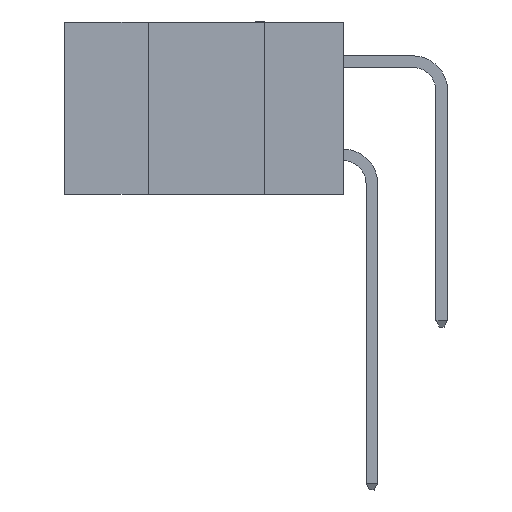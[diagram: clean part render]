
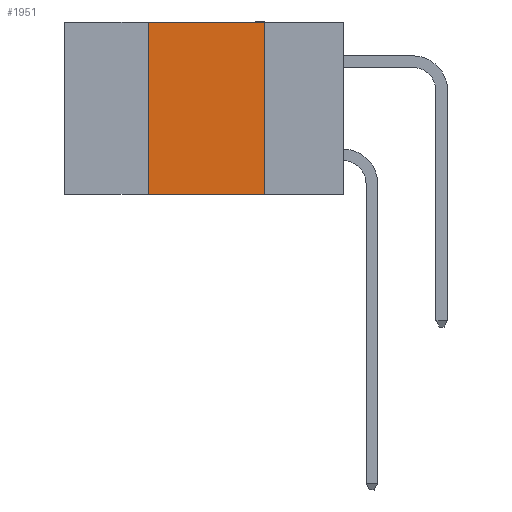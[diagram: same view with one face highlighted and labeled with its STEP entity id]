
A CAD part, left-side view. The second image highlights one B-rep face of the part: STEP entity #1951.
In plain terms, the highlighted planar face has unit normal (-1, 0, 0).
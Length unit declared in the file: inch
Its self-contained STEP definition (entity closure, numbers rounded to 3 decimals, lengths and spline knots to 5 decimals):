
#231 = CARTESIAN_POINT ( 'NONE',  ( 0., 0.42, -0.37 ) ) ;
#1951 = ADVANCED_FACE ( 'NONE', ( #21631 ), #26591, .F. ) ;
#3269 = DIRECTION ( 'NONE',  ( 1., 0., 0. ) ) ;
#3896 = EDGE_CURVE ( 'NONE', #22698, #11320, #11209, .T. ) ;
#4561 = ORIENTED_EDGE ( 'NONE', *, *, #11074, .F. ) ;
#5219 = DIRECTION ( 'NONE',  ( 0., 0., -1. ) ) ;
#5427 = DIRECTION ( 'NONE',  ( 0., 0., -1. ) ) ;
#6003 = CARTESIAN_POINT ( 'NONE',  ( 0., 0.17, -0.37 ) ) ;
#6651 = ORIENTED_EDGE ( 'NONE', *, *, #8108, .F. ) ;
#7099 = LINE ( 'NONE', #7462, #9716 ) ;
#7162 = ORIENTED_EDGE ( 'NONE', *, *, #3896, .T. ) ;
#7462 = CARTESIAN_POINT ( 'NONE',  ( 0., 0.6, 0. ) ) ;
#8108 = EDGE_CURVE ( 'NONE', #22698, #24449, #14214, .T. ) ;
#9568 = DIRECTION ( 'NONE',  ( 0., -1., 0. ) ) ;
#9716 = VECTOR ( 'NONE', #9568, 39.37008 ) ;
#10624 = VECTOR ( 'NONE', #5427, 39.37008 ) ;
#10855 = CARTESIAN_POINT ( 'NONE',  ( 0., 0.6, -0.37 ) ) ;
#11074 = EDGE_CURVE ( 'NONE', #24449, #17799, #7099, .T. ) ;
#11209 = LINE ( 'NONE', #10855, #22180 ) ;
#11320 = VERTEX_POINT ( 'NONE', #6003 ) ;
#11973 = CARTESIAN_POINT ( 'NONE',  ( 0., 0.17, 0. ) ) ;
#12795 = EDGE_LOOP ( 'NONE', ( #14413, #4561, #6651, #7162 ) ) ;
#13287 = LINE ( 'NONE', #11973, #10624 ) ;
#14214 = LINE ( 'NONE', #14961, #22496 ) ;
#14413 = ORIENTED_EDGE ( 'NONE', *, *, #22510, .F. ) ;
#14961 = CARTESIAN_POINT ( 'NONE',  ( 0., 0.42, 0. ) ) ;
#17406 = DIRECTION ( 'NONE',  ( 0., -1., 0. ) ) ;
#17799 = VERTEX_POINT ( 'NONE', #25397 ) ;
#21631 = FACE_OUTER_BOUND ( 'NONE', #12795, .T. ) ;
#22180 = VECTOR ( 'NONE', #17406, 39.37008 ) ;
#22496 = VECTOR ( 'NONE', #23495, 39.37008 ) ;
#22510 = EDGE_CURVE ( 'NONE', #17799, #11320, #13287, .T. ) ;
#22557 = CARTESIAN_POINT ( 'NONE',  ( 0., 0.42, 0. ) ) ;
#22698 = VERTEX_POINT ( 'NONE', #231 ) ;
#23495 = DIRECTION ( 'NONE',  ( 0., 0., 1. ) ) ;
#23632 = AXIS2_PLACEMENT_3D ( 'NONE', #26497, #3269, #5219 ) ;
#24449 = VERTEX_POINT ( 'NONE', #22557 ) ;
#25397 = CARTESIAN_POINT ( 'NONE',  ( 0., 0.17, 0. ) ) ;
#26497 = CARTESIAN_POINT ( 'NONE',  ( 0., 0.6, 0. ) ) ;
#26591 = PLANE ( 'NONE',  #23632 ) ;
